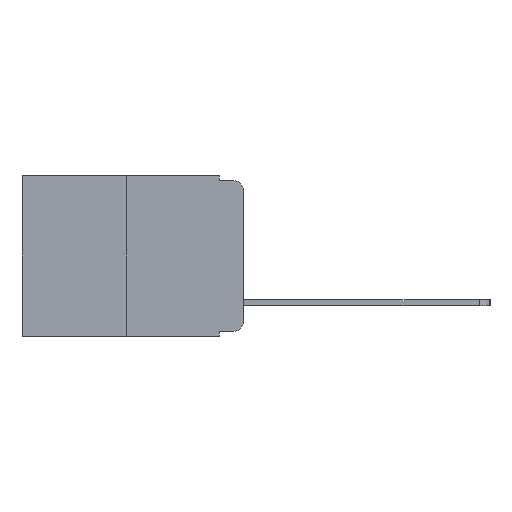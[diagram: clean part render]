
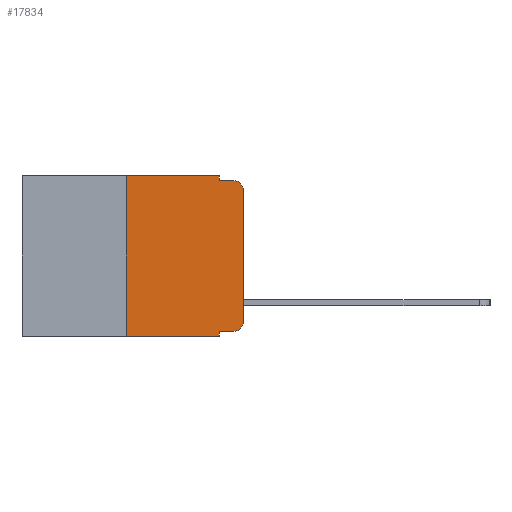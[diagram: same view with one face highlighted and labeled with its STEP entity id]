
A CAD part, left-side view. The second image highlights one B-rep face of the part: STEP entity #17834.
In plain terms, the highlighted planar face has unit normal (-1, 0, 0).
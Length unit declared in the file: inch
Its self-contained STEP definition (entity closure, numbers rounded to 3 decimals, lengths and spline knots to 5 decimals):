
#307 = CARTESIAN_POINT ( 'NONE',  ( 0., 0.473, 0. ) ) ;
#687 = VECTOR ( 'NONE', #15109, 39.37008 ) ;
#699 = VERTEX_POINT ( 'NONE', #16403 ) ;
#1238 = EDGE_CURVE ( 'NONE', #9401, #8604, #5658, .T. ) ;
#1401 = CARTESIAN_POINT ( 'NONE',  ( 0., 0.051, -0.343 ) ) ;
#1627 = ORIENTED_EDGE ( 'NONE', *, *, #7765, .F. ) ;
#1939 = DIRECTION ( 'NONE',  ( 1., 0., 0. ) ) ;
#1974 = DIRECTION ( 'NONE',  ( 0., 0., 1. ) ) ;
#2318 = VECTOR ( 'NONE', #8622, 39.37008 ) ;
#2561 = CARTESIAN_POINT ( 'NONE',  ( 0., 0.02, -0.313 ) ) ;
#3766 = CARTESIAN_POINT ( 'NONE',  ( 0., 0.473, 0. ) ) ;
#4083 = DIRECTION ( 'NONE',  ( 0., 0., -1. ) ) ;
#4362 = EDGE_CURVE ( 'NONE', #12113, #6144, #6280, .T. ) ;
#4400 = CARTESIAN_POINT ( 'NONE',  ( 0., 0., -0.03 ) ) ;
#4810 = LINE ( 'NONE', #12698, #12261 ) ;
#4851 = LINE ( 'NONE', #9176, #687 ) ;
#4891 = CARTESIAN_POINT ( 'NONE',  ( 0., 0., -0.313 ) ) ;
#5014 = CARTESIAN_POINT ( 'NONE',  ( 0., 0.25, 0. ) ) ;
#5134 = LINE ( 'NONE', #6259, #12561 ) ;
#5187 = AXIS2_PLACEMENT_3D ( 'NONE', #307, #1939, #12460 ) ;
#5247 = VERTEX_POINT ( 'NONE', #4400 ) ;
#5658 = LINE ( 'NONE', #13530, #13056 ) ;
#6144 = VERTEX_POINT ( 'NONE', #9868 ) ;
#6259 = CARTESIAN_POINT ( 'NONE',  ( 0., 0.051, -0.333 ) ) ;
#6280 = LINE ( 'NONE', #7036, #17476 ) ;
#6312 = VERTEX_POINT ( 'NONE', #4891 ) ;
#6316 = EDGE_LOOP ( 'NONE', ( #14209, #14643, #15411, #15018, #15812, #13153, #10257, #1627, #19166, #12476 ) ) ;
#6350 = DIRECTION ( 'NONE',  ( -1., 0., 0. ) ) ;
#6559 = PLANE ( 'NONE',  #5187 ) ;
#7036 = CARTESIAN_POINT ( 'NONE',  ( 0., 0.051, -0.01 ) ) ;
#7159 = CARTESIAN_POINT ( 'NONE',  ( 0., 0.051, 0. ) ) ;
#7765 = EDGE_CURVE ( 'NONE', #7788, #8604, #4810, .T. ) ;
#7788 = VERTEX_POINT ( 'NONE', #18518 ) ;
#8604 = VERTEX_POINT ( 'NONE', #1401 ) ;
#8622 = DIRECTION ( 'NONE',  ( 0., 0., -1. ) ) ;
#9176 = CARTESIAN_POINT ( 'NONE',  ( 0., 0., 0. ) ) ;
#9401 = VERTEX_POINT ( 'NONE', #15250 ) ;
#9456 = EDGE_CURVE ( 'NONE', #9401, #11499, #17225, .T. ) ;
#9567 = EDGE_CURVE ( 'NONE', #11499, #699, #19144, .T. ) ;
#9734 = DIRECTION ( 'NONE',  ( 0., 0., -1. ) ) ;
#9868 = CARTESIAN_POINT ( 'NONE',  ( 0., 0.02, -0.01 ) ) ;
#10248 = CIRCLE ( 'NONE', #11640, 0.02 ) ;
#10257 = ORIENTED_EDGE ( 'NONE', *, *, #1238, .T. ) ;
#11499 = VERTEX_POINT ( 'NONE', #18899 ) ;
#11640 = AXIS2_PLACEMENT_3D ( 'NONE', #2561, #13045, #4083 ) ;
#12113 = VERTEX_POINT ( 'NONE', #17550 ) ;
#12261 = VECTOR ( 'NONE', #9734, 39.37008 ) ;
#12460 = DIRECTION ( 'NONE',  ( 0., 0., -1. ) ) ;
#12476 = ORIENTED_EDGE ( 'NONE', *, *, #14580, .T. ) ;
#12561 = VECTOR ( 'NONE', #15059, 39.37008 ) ;
#12698 = CARTESIAN_POINT ( 'NONE',  ( 0., 0.051, 0. ) ) ;
#13045 = DIRECTION ( 'NONE',  ( -1., 0., 0. ) ) ;
#13056 = VECTOR ( 'NONE', #16675, 39.37008 ) ;
#13153 = ORIENTED_EDGE ( 'NONE', *, *, #9456, .F. ) ;
#13366 = VECTOR ( 'NONE', #1974, 39.37008 ) ;
#13530 = CARTESIAN_POINT ( 'NONE',  ( 0., 0.473, -0.343 ) ) ;
#13613 = EDGE_CURVE ( 'NONE', #7788, #14457, #5134, .T. ) ;
#14197 = DIRECTION ( 'NONE',  ( 0., -1., 0. ) ) ;
#14209 = ORIENTED_EDGE ( 'NONE', *, *, #14214, .T. ) ;
#14214 = EDGE_CURVE ( 'NONE', #6312, #5247, #4851, .T. ) ;
#14228 = LINE ( 'NONE', #7159, #2318 ) ;
#14457 = VERTEX_POINT ( 'NONE', #15678 ) ;
#14580 = EDGE_CURVE ( 'NONE', #14457, #6312, #10248, .T. ) ;
#14643 = ORIENTED_EDGE ( 'NONE', *, *, #15219, .T. ) ;
#14719 = FACE_OUTER_BOUND ( 'NONE', #6316, .T. ) ;
#15018 = ORIENTED_EDGE ( 'NONE', *, *, #18503, .F. ) ;
#15059 = DIRECTION ( 'NONE',  ( 0., -1., 0. ) ) ;
#15109 = DIRECTION ( 'NONE',  ( 0., 0., 1. ) ) ;
#15160 = CARTESIAN_POINT ( 'NONE',  ( 0., 0.02, -0.03 ) ) ;
#15219 = EDGE_CURVE ( 'NONE', #5247, #6144, #18967, .T. ) ;
#15250 = CARTESIAN_POINT ( 'NONE',  ( 0., 0.25, -0.343 ) ) ;
#15411 = ORIENTED_EDGE ( 'NONE', *, *, #4362, .F. ) ;
#15446 = VECTOR ( 'NONE', #14197, 39.37008 ) ;
#15678 = CARTESIAN_POINT ( 'NONE',  ( 0., 0.02, -0.333 ) ) ;
#15812 = ORIENTED_EDGE ( 'NONE', *, *, #9567, .F. ) ;
#16403 = CARTESIAN_POINT ( 'NONE',  ( 0., 0.051, 0. ) ) ;
#16616 = DIRECTION ( 'NONE',  ( 0., 0., -1. ) ) ;
#16675 = DIRECTION ( 'NONE',  ( 0., -1., 0. ) ) ;
#16777 = AXIS2_PLACEMENT_3D ( 'NONE', #15160, #6350, #16616 ) ;
#17225 = LINE ( 'NONE', #5014, #13366 ) ;
#17476 = VECTOR ( 'NONE', #18596, 39.37008 ) ;
#17550 = CARTESIAN_POINT ( 'NONE',  ( 0., 0.051, -0.01 ) ) ;
#17834 = ADVANCED_FACE ( 'NONE', ( #14719 ), #6559, .F. ) ;
#18503 = EDGE_CURVE ( 'NONE', #699, #12113, #14228, .T. ) ;
#18518 = CARTESIAN_POINT ( 'NONE',  ( 0., 0.051, -0.333 ) ) ;
#18596 = DIRECTION ( 'NONE',  ( 0., -1., 0. ) ) ;
#18899 = CARTESIAN_POINT ( 'NONE',  ( 0., 0.25, 0. ) ) ;
#18967 = CIRCLE ( 'NONE', #16777, 0.02 ) ;
#19144 = LINE ( 'NONE', #3766, #15446 ) ;
#19166 = ORIENTED_EDGE ( 'NONE', *, *, #13613, .T. ) ;
